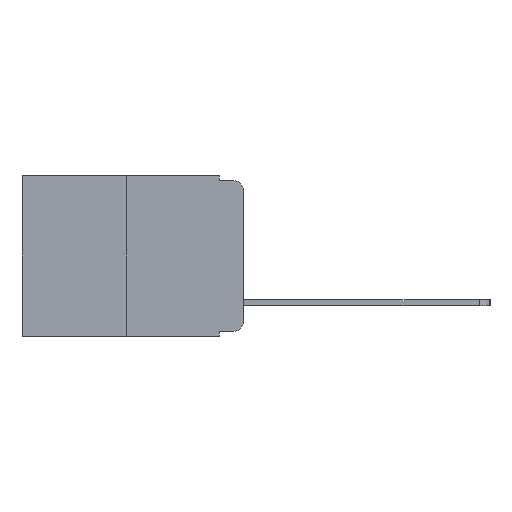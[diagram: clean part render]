
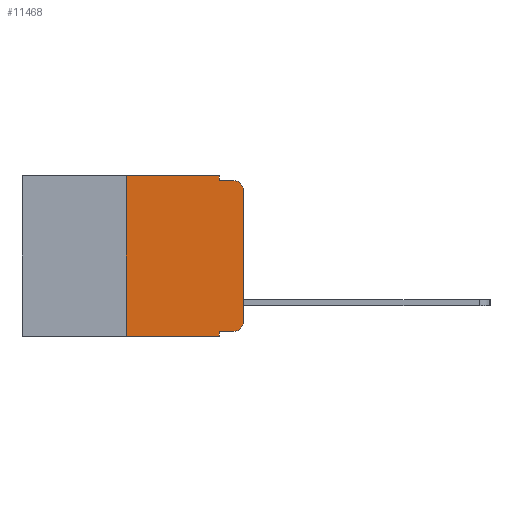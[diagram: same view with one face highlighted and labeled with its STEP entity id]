
A CAD part, left-side view. The second image highlights one B-rep face of the part: STEP entity #11468.
In plain terms, the highlighted planar face has unit normal (-1, 0, 0).
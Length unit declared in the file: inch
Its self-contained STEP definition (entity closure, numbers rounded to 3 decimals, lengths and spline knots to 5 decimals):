
#253 = ORIENTED_EDGE ( 'NONE', *, *, #10132, .F. ) ;
#254 = EDGE_CURVE ( 'NONE', #5505, #1133, #2971, .T. ) ;
#386 = DIRECTION ( 'NONE',  ( 0., -1., 0. ) ) ;
#448 = LINE ( 'NONE', #11236, #2943 ) ;
#604 = ORIENTED_EDGE ( 'NONE', *, *, #1601, .F. ) ;
#632 = VECTOR ( 'NONE', #3696, 39.37008 ) ;
#872 = VERTEX_POINT ( 'NONE', #11645 ) ;
#952 = DIRECTION ( 'NONE',  ( 0., 0., -1. ) ) ;
#971 = VECTOR ( 'NONE', #4119, 39.37008 ) ;
#1001 = EDGE_CURVE ( 'NONE', #5804, #5505, #2648, .T. ) ;
#1051 = DIRECTION ( 'NONE',  ( 0., 0., -1. ) ) ;
#1133 = VERTEX_POINT ( 'NONE', #5902 ) ;
#1197 = VERTEX_POINT ( 'NONE', #1806 ) ;
#1200 = CARTESIAN_POINT ( 'NONE',  ( 0., 0.02, -0.333 ) ) ;
#1209 = EDGE_LOOP ( 'NONE', ( #11879, #12197, #4579, #253, #604, #3737, #4098, #7242, #10310, #13313 ) ) ;
#1590 = DIRECTION ( 'NONE',  ( 0., 0., -1. ) ) ;
#1601 = EDGE_CURVE ( 'NONE', #8989, #872, #9371, .T. ) ;
#1793 = DIRECTION ( 'NONE',  ( 0., 0., 1. ) ) ;
#1794 = FACE_OUTER_BOUND ( 'NONE', #1209, .T. ) ;
#1806 = CARTESIAN_POINT ( 'NONE',  ( 0., 0.25, -0.343 ) ) ;
#2087 = CARTESIAN_POINT ( 'NONE',  ( 0., 0.473, -0.343 ) ) ;
#2507 = VERTEX_POINT ( 'NONE', #10475 ) ;
#2648 = LINE ( 'NONE', #8842, #5444 ) ;
#2840 = CARTESIAN_POINT ( 'NONE',  ( 0., 0.25, 0. ) ) ;
#2880 = DIRECTION ( 'NONE',  ( 0., 0., -1. ) ) ;
#2943 = VECTOR ( 'NONE', #2880, 39.37008 ) ;
#2971 = CIRCLE ( 'NONE', #4303, 0.02 ) ;
#3565 = CIRCLE ( 'NONE', #7063, 0.02 ) ;
#3646 = EDGE_CURVE ( 'NONE', #1197, #2507, #10265, .T. ) ;
#3696 = DIRECTION ( 'NONE',  ( 0., -1., 0. ) ) ;
#3737 = ORIENTED_EDGE ( 'NONE', *, *, #7377, .F. ) ;
#3767 = LINE ( 'NONE', #10379, #971 ) ;
#4098 = ORIENTED_EDGE ( 'NONE', *, *, #3646, .T. ) ;
#4119 = DIRECTION ( 'NONE',  ( 0., -1., 0. ) ) ;
#4303 = AXIS2_PLACEMENT_3D ( 'NONE', #4503, #11749, #5551 ) ;
#4411 = VERTEX_POINT ( 'NONE', #12774 ) ;
#4501 = VERTEX_POINT ( 'NONE', #6778 ) ;
#4503 = CARTESIAN_POINT ( 'NONE',  ( 0., 0.02, -0.313 ) ) ;
#4540 = EDGE_CURVE ( 'NONE', #5804, #2507, #5072, .T. ) ;
#4579 = ORIENTED_EDGE ( 'NONE', *, *, #10826, .F. ) ;
#4707 = VECTOR ( 'NONE', #13454, 39.37008 ) ;
#4931 = AXIS2_PLACEMENT_3D ( 'NONE', #9326, #7298, #952 ) ;
#5072 = LINE ( 'NONE', #7929, #10623 ) ;
#5165 = DIRECTION ( 'NONE',  ( 0., 0., 1. ) ) ;
#5444 = VECTOR ( 'NONE', #386, 39.37008 ) ;
#5505 = VERTEX_POINT ( 'NONE', #1200 ) ;
#5551 = DIRECTION ( 'NONE',  ( 0., 0., -1. ) ) ;
#5708 = VERTEX_POINT ( 'NONE', #7809 ) ;
#5804 = VERTEX_POINT ( 'NONE', #9010 ) ;
#5885 = LINE ( 'NONE', #10378, #6560 ) ;
#5902 = CARTESIAN_POINT ( 'NONE',  ( 0., 0., -0.313 ) ) ;
#6560 = VECTOR ( 'NONE', #5165, 39.37008 ) ;
#6778 = CARTESIAN_POINT ( 'NONE',  ( 0., 0.051, -0.01 ) ) ;
#7063 = AXIS2_PLACEMENT_3D ( 'NONE', #13486, #7380, #1051 ) ;
#7242 = ORIENTED_EDGE ( 'NONE', *, *, #4540, .F. ) ;
#7298 = DIRECTION ( 'NONE',  ( 1., 0., 0. ) ) ;
#7377 = EDGE_CURVE ( 'NONE', #1197, #8989, #11339, .T. ) ;
#7380 = DIRECTION ( 'NONE',  ( -1., 0., 0. ) ) ;
#7809 = CARTESIAN_POINT ( 'NONE',  ( 0., 0., -0.03 ) ) ;
#7929 = CARTESIAN_POINT ( 'NONE',  ( 0., 0.051, 0. ) ) ;
#8141 = CARTESIAN_POINT ( 'NONE',  ( 0., 0.25, 0. ) ) ;
#8781 = CARTESIAN_POINT ( 'NONE',  ( 0., 0.473, 0. ) ) ;
#8842 = CARTESIAN_POINT ( 'NONE',  ( 0., 0.051, -0.333 ) ) ;
#8989 = VERTEX_POINT ( 'NONE', #8141 ) ;
#9010 = CARTESIAN_POINT ( 'NONE',  ( 0., 0.051, -0.333 ) ) ;
#9266 = VECTOR ( 'NONE', #1793, 39.37008 ) ;
#9326 = CARTESIAN_POINT ( 'NONE',  ( 0., 0.473, 0. ) ) ;
#9371 = LINE ( 'NONE', #8781, #632 ) ;
#10132 = EDGE_CURVE ( 'NONE', #872, #4501, #448, .T. ) ;
#10265 = LINE ( 'NONE', #2087, #4707 ) ;
#10310 = ORIENTED_EDGE ( 'NONE', *, *, #1001, .T. ) ;
#10378 = CARTESIAN_POINT ( 'NONE',  ( 0., 0., 0. ) ) ;
#10379 = CARTESIAN_POINT ( 'NONE',  ( 0., 0.051, -0.01 ) ) ;
#10475 = CARTESIAN_POINT ( 'NONE',  ( 0., 0.051, -0.343 ) ) ;
#10623 = VECTOR ( 'NONE', #1590, 39.37008 ) ;
#10826 = EDGE_CURVE ( 'NONE', #4501, #4411, #3767, .T. ) ;
#11236 = CARTESIAN_POINT ( 'NONE',  ( 0., 0.051, 0. ) ) ;
#11339 = LINE ( 'NONE', #2840, #9266 ) ;
#11379 = PLANE ( 'NONE',  #4931 ) ;
#11468 = ADVANCED_FACE ( 'NONE', ( #1794 ), #11379, .F. ) ;
#11504 = EDGE_CURVE ( 'NONE', #5708, #4411, #3565, .T. ) ;
#11645 = CARTESIAN_POINT ( 'NONE',  ( 0., 0.051, 0. ) ) ;
#11749 = DIRECTION ( 'NONE',  ( -1., 0., 0. ) ) ;
#11879 = ORIENTED_EDGE ( 'NONE', *, *, #12176, .T. ) ;
#12176 = EDGE_CURVE ( 'NONE', #1133, #5708, #5885, .T. ) ;
#12197 = ORIENTED_EDGE ( 'NONE', *, *, #11504, .T. ) ;
#12774 = CARTESIAN_POINT ( 'NONE',  ( 0., 0.02, -0.01 ) ) ;
#13313 = ORIENTED_EDGE ( 'NONE', *, *, #254, .T. ) ;
#13454 = DIRECTION ( 'NONE',  ( 0., -1., 0. ) ) ;
#13486 = CARTESIAN_POINT ( 'NONE',  ( 0., 0.02, -0.03 ) ) ;
